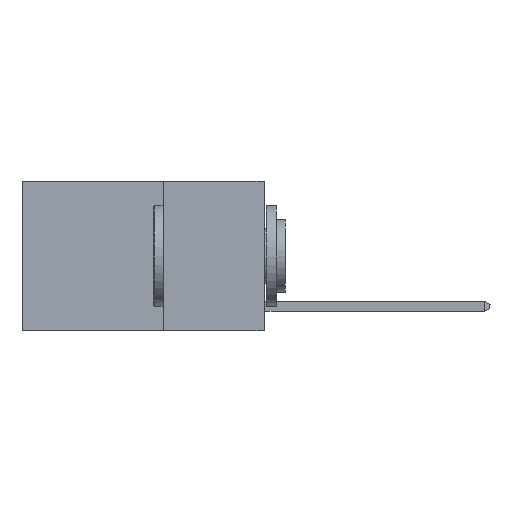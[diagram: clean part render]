
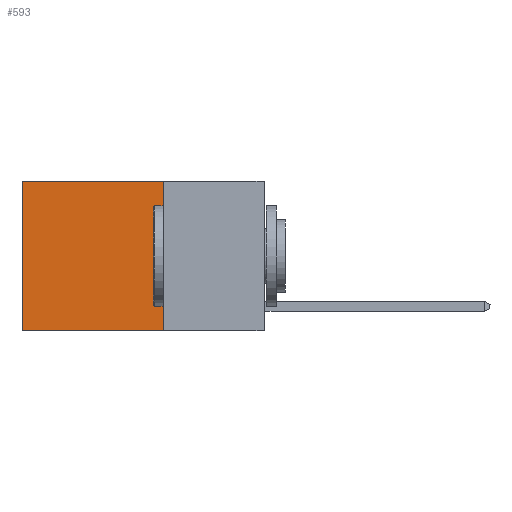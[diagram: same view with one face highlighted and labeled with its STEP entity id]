
A CAD part, left-side view. The second image highlights one B-rep face of the part: STEP entity #593.
In plain terms, the highlighted planar face has unit normal (-1, 0, 0).
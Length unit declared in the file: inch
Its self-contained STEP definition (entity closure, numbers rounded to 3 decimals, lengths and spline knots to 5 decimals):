
#593 = ADVANCED_FACE ( 'NONE', ( #15188 ), #13768, .F. ) ;
#803 = CARTESIAN_POINT ( 'NONE',  ( 0.2625, 0.6, -0.37 ) ) ;
#1660 = LINE ( 'NONE', #14223, #11926 ) ;
#1662 = CARTESIAN_POINT ( 'NONE',  ( 0.2625, 0.25, 0. ) ) ;
#2400 = DIRECTION ( 'NONE',  ( 0., 0., -1. ) ) ;
#2566 = DIRECTION ( 'NONE',  ( 0., 1., 0. ) ) ;
#4634 = EDGE_LOOP ( 'NONE', ( #5836, #18798, #7904, #11896 ) ) ;
#5014 = VERTEX_POINT ( 'NONE', #12822 ) ;
#5289 = EDGE_CURVE ( 'NONE', #15015, #5014, #14062, .T. ) ;
#5836 = ORIENTED_EDGE ( 'NONE', *, *, #6274, .T. ) ;
#6213 = CARTESIAN_POINT ( 'NONE',  ( 0.2625, 0.25, 0. ) ) ;
#6274 = EDGE_CURVE ( 'NONE', #5014, #18192, #10727, .T. ) ;
#6753 = CARTESIAN_POINT ( 'NONE',  ( 0.2625, 0.25, 0. ) ) ;
#6803 = VECTOR ( 'NONE', #2400, 39.37008 ) ;
#7674 = DIRECTION ( 'NONE',  ( 0., 1., 0. ) ) ;
#7904 = ORIENTED_EDGE ( 'NONE', *, *, #16955, .F. ) ;
#8953 = AXIS2_PLACEMENT_3D ( 'NONE', #13766, #13705, #13699 ) ;
#9753 = VECTOR ( 'NONE', #7674, 39.37008 ) ;
#9930 = VERTEX_POINT ( 'NONE', #15240 ) ;
#10727 = LINE ( 'NONE', #16105, #18088 ) ;
#11641 = DIRECTION ( 'NONE',  ( 0., 0., -1. ) ) ;
#11896 = ORIENTED_EDGE ( 'NONE', *, *, #5289, .T. ) ;
#11926 = VECTOR ( 'NONE', #2566, 39.37008 ) ;
#12822 = CARTESIAN_POINT ( 'NONE',  ( 0.2625, 0.6, 0. ) ) ;
#12846 = EDGE_CURVE ( 'NONE', #9930, #18192, #1660, .T. ) ;
#13699 = DIRECTION ( 'NONE',  ( 0., 0., -1. ) ) ;
#13705 = DIRECTION ( 'NONE',  ( 1., 0., 0. ) ) ;
#13766 = CARTESIAN_POINT ( 'NONE',  ( 0.2625, 0.25, 0. ) ) ;
#13768 = PLANE ( 'NONE',  #8953 ) ;
#14062 = LINE ( 'NONE', #6213, #9753 ) ;
#14072 = LINE ( 'NONE', #6753, #6803 ) ;
#14223 = CARTESIAN_POINT ( 'NONE',  ( 0.2625, 0.25, -0.37 ) ) ;
#15015 = VERTEX_POINT ( 'NONE', #1662 ) ;
#15188 = FACE_OUTER_BOUND ( 'NONE', #4634, .T. ) ;
#15240 = CARTESIAN_POINT ( 'NONE',  ( 0.2625, 0.25, -0.37 ) ) ;
#16105 = CARTESIAN_POINT ( 'NONE',  ( 0.2625, 0.6, 0. ) ) ;
#16955 = EDGE_CURVE ( 'NONE', #15015, #9930, #14072, .T. ) ;
#18088 = VECTOR ( 'NONE', #11641, 39.37008 ) ;
#18192 = VERTEX_POINT ( 'NONE', #803 ) ;
#18798 = ORIENTED_EDGE ( 'NONE', *, *, #12846, .F. ) ;
